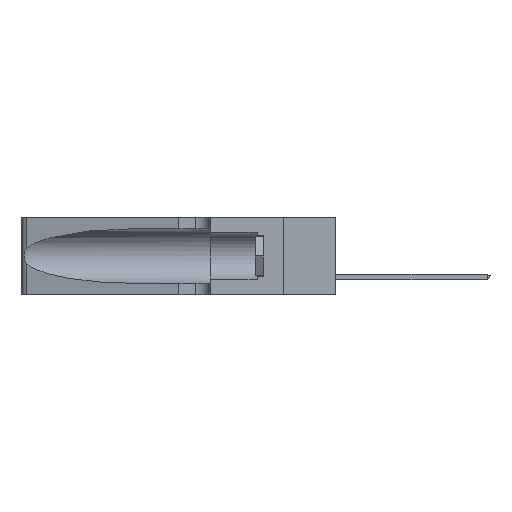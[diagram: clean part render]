
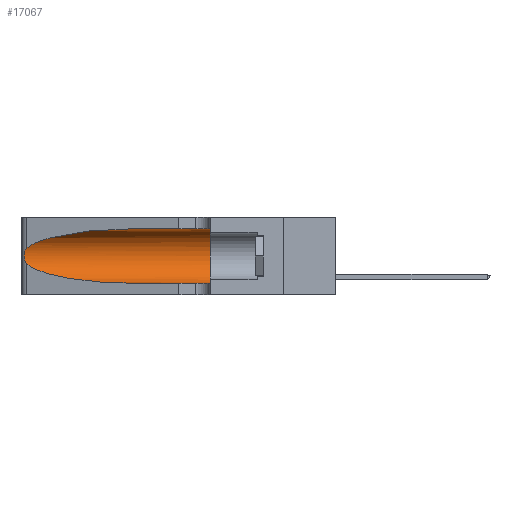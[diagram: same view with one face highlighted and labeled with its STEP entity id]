
A CAD part, left-side view. The second image highlights one B-rep face of the part: STEP entity #17067.
In plain terms, the highlighted cylindrical face has radius 3.308 mm (diameter 6.617 mm), a partial arc.
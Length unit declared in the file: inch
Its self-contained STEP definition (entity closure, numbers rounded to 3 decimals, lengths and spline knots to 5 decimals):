
#47 = AXIS2_PLACEMENT_3D ( 'NONE', #24035, #27090, #10485 ) ;
#589 = FACE_OUTER_BOUND ( 'NONE', #12083, .T. ) ;
#835 = DIRECTION ( 'NONE',  ( 0., -1., 0. ) ) ;
#849 = VERTEX_POINT ( 'NONE', #1188 ) ;
#1182 = CARTESIAN_POINT ( 'NONE',  ( 0.25639, 1.23184, 0.21858 ) ) ;
#1188 = CARTESIAN_POINT ( 'NONE',  ( 0.1305, 0.72297, 0.05475 ) ) ;
#2576 = LINE ( 'NONE', #28573, #27711 ) ;
#2837 = CARTESIAN_POINT ( 'NONE',  ( 0.1305, 0.72297, 0.31525 ) ) ;
#3593 =( BOUNDED_CURVE ( )  B_SPLINE_CURVE ( 3, ( #39148, #8480, #15323, #39310 ),
 .UNSPECIFIED., .F., .F. ) 
 B_SPLINE_CURVE_WITH_KNOTS ( ( 4, 4 ),
 ( 1.5708, 2.84003 ),
 .UNSPECIFIED. ) 
 CURVE ( )  GEOMETRIC_REPRESENTATION_ITEM ( )  RATIONAL_B_SPLINE_CURVE ( ( 1., 0.87, 0.87, 1. ) ) 
 REPRESENTATION_ITEM ( '' )  );
#3807 = VERTEX_POINT ( 'NONE', #37982 ) ;
#4243 = DIRECTION ( 'NONE',  ( 0., -1., 0. ) ) ;
#4523 = CARTESIAN_POINT ( 'NONE',  ( 0.26075, 1.23896, 0.178 ) ) ;
#5004 = CYLINDRICAL_SURFACE ( 'NONE', #18274, 0.13025 ) ;
#5491 = CARTESIAN_POINT ( 'NONE',  ( 0.25639, 1.23186, 0.15144 ) ) ;
#7822 = CARTESIAN_POINT ( 'NONE',  ( 0.25854, 1.2359, 0.20912 ) ) ;
#7979 = CARTESIAN_POINT ( 'NONE',  ( 0.26017, 1.23833, 0.17102 ) ) ;
#8480 = CARTESIAN_POINT ( 'NONE',  ( 0.18966, 0.96281, 0.31525 ) ) ;
#8792 = CARTESIAN_POINT ( 'NONE',  ( 0.25487, 1.22718, 0.14631 ) ) ;
#8817 = ORIENTED_EDGE ( 'NONE', *, *, #42937, .T. ) ;
#10212 = LINE ( 'NONE', #21118, #39609 ) ;
#10485 = DIRECTION ( 'NONE',  ( 0., 0., 1. ) ) ;
#11325 = CARTESIAN_POINT ( 'NONE',  ( 0.26075, 1.23896, 0.19203 ) ) ;
#12083 = EDGE_LOOP ( 'NONE', ( #13031, #24047, #8817, #16313, #14987, #13705 ) ) ;
#12495 = EDGE_CURVE ( 'NONE', #40071, #20801, #10212, .T. ) ;
#12634 = CARTESIAN_POINT ( 'NONE',  ( 0.18966, 0.96281, 0.05475 ) ) ;
#13031 = ORIENTED_EDGE ( 'NONE', *, *, #40470, .T. ) ;
#13705 = ORIENTED_EDGE ( 'NONE', *, *, #12495, .F. ) ;
#14143 = DIRECTION ( 'NONE',  ( 0., -1., 0. ) ) ;
#14987 = ORIENTED_EDGE ( 'NONE', *, *, #30448, .F. ) ;
#15300 = CARTESIAN_POINT ( 'NONE',  ( 0.25787, 1.23484, 0.2124 ) ) ;
#15323 = CARTESIAN_POINT ( 'NONE',  ( 0.2373, 1.15595, 0.28018 ) ) ;
#15379 =( BOUNDED_CURVE ( )  B_SPLINE_CURVE ( 3, ( #19729, #33698, #12634, #19446 ),
 .UNSPECIFIED., .F., .F. ) 
 B_SPLINE_CURVE_WITH_KNOTS ( ( 4, 4 ),
 ( 3.44316, 4.71239 ),
 .UNSPECIFIED. ) 
 CURVE ( )  GEOMETRIC_REPRESENTATION_ITEM ( )  RATIONAL_B_SPLINE_CURVE ( ( 1., 0.87, 0.87, 1. ) ) 
 REPRESENTATION_ITEM ( '' )  );
#16069 = CARTESIAN_POINT ( 'NONE',  ( 0.25555, 1.22993, 0.14849 ) ) ;
#16313 = ORIENTED_EDGE ( 'NONE', *, *, #37502, .T. ) ;
#17067 = ADVANCED_FACE ( 'NONE', ( #589 ), #5004, .F. ) ;
#18274 = AXIS2_PLACEMENT_3D ( 'NONE', #25033, #4243, #38519 ) ;
#18883 = VERTEX_POINT ( 'NONE', #36746 ) ;
#19446 = CARTESIAN_POINT ( 'NONE',  ( 0.1305, 0.72297, 0.05475 ) ) ;
#19729 = CARTESIAN_POINT ( 'NONE',  ( 0.25487, 1.22718, 0.14631 ) ) ;
#20801 = VERTEX_POINT ( 'NONE', #35114 ) ;
#21118 = CARTESIAN_POINT ( 'NONE',  ( 0.1305, 1.61858, 0.31525 ) ) ;
#22822 = B_SPLINE_CURVE_WITH_KNOTS ( 'NONE', 3,
 ( #25006, #35796, #1182, #15300, #7822, #31765, #11325, #4523, #7979, #32066, #31925, #5491, #16069, #8792 ),
 .UNSPECIFIED., .F., .F.,
 ( 4, 2, 2, 2, 2, 2, 4 ),
 ( 0., 0.00027, 0.00053, 0.00107, 0.0016, 0.00187, 0.00214 ),
 .UNSPECIFIED. ) ;
#24035 = CARTESIAN_POINT ( 'NONE',  ( 0.1305, 0.35, 0.185 ) ) ;
#24047 = ORIENTED_EDGE ( 'NONE', *, *, #37920, .T. ) ;
#25006 = CARTESIAN_POINT ( 'NONE',  ( 0.25487, 1.22718, 0.22369 ) ) ;
#25033 = CARTESIAN_POINT ( 'NONE',  ( 0.1305, 1.61858, 0.185 ) ) ;
#25286 = CIRCLE ( 'NONE', #47, 0.13025 ) ;
#27090 = DIRECTION ( 'NONE',  ( 0., 1., 0. ) ) ;
#27711 = VECTOR ( 'NONE', #835, 39.37008 ) ;
#28573 = CARTESIAN_POINT ( 'NONE',  ( 0.1305, 1.61858, 0.05475 ) ) ;
#30448 = EDGE_CURVE ( 'NONE', #20801, #36332, #25286, .T. ) ;
#31765 = CARTESIAN_POINT ( 'NONE',  ( 0.26018, 1.23835, 0.19895 ) ) ;
#31925 = CARTESIAN_POINT ( 'NONE',  ( 0.25789, 1.23486, 0.15765 ) ) ;
#32066 = CARTESIAN_POINT ( 'NONE',  ( 0.25856, 1.23593, 0.16098 ) ) ;
#33698 = CARTESIAN_POINT ( 'NONE',  ( 0.2373, 1.15595, 0.08982 ) ) ;
#35114 = CARTESIAN_POINT ( 'NONE',  ( 0.1305, 0.35, 0.31525 ) ) ;
#35796 = CARTESIAN_POINT ( 'NONE',  ( 0.25555, 1.22994, 0.2215 ) ) ;
#36332 = VERTEX_POINT ( 'NONE', #44026 ) ;
#36746 = CARTESIAN_POINT ( 'NONE',  ( 0.25487, 1.22718, 0.22369 ) ) ;
#37502 = EDGE_CURVE ( 'NONE', #849, #36332, #2576, .T. ) ;
#37920 = EDGE_CURVE ( 'NONE', #18883, #3807, #22822, .T. ) ;
#37982 = CARTESIAN_POINT ( 'NONE',  ( 0.25487, 1.22718, 0.14631 ) ) ;
#38519 = DIRECTION ( 'NONE',  ( 0., 0., -1. ) ) ;
#39148 = CARTESIAN_POINT ( 'NONE',  ( 0.1305, 0.72297, 0.31525 ) ) ;
#39310 = CARTESIAN_POINT ( 'NONE',  ( 0.25487, 1.22718, 0.22369 ) ) ;
#39609 = VECTOR ( 'NONE', #14143, 39.37008 ) ;
#40071 = VERTEX_POINT ( 'NONE', #2837 ) ;
#40470 = EDGE_CURVE ( 'NONE', #40071, #18883, #3593, .T. ) ;
#42937 = EDGE_CURVE ( 'NONE', #3807, #849, #15379, .T. ) ;
#44026 = CARTESIAN_POINT ( 'NONE',  ( 0.1305, 0.35, 0.05475 ) ) ;
